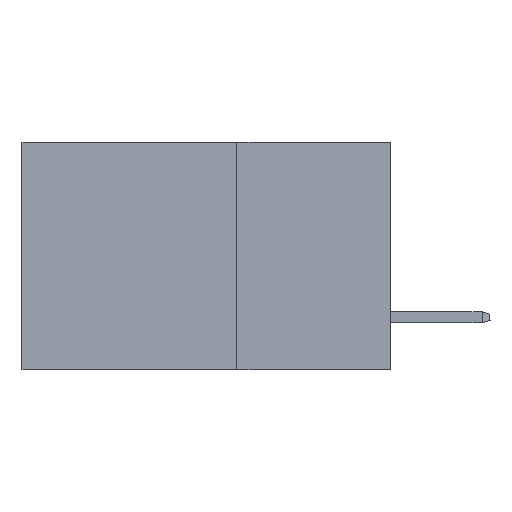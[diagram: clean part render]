
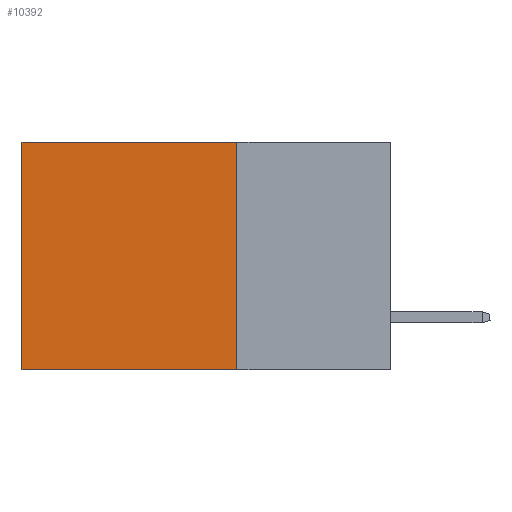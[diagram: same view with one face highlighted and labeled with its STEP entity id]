
A CAD part, left-side view. The second image highlights one B-rep face of the part: STEP entity #10392.
In plain terms, the highlighted planar face has unit normal (-1, 0, 0).
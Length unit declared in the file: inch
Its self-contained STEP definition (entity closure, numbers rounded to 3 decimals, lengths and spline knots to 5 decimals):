
#921 = DIRECTION ( 'NONE',  ( 0., 1., 0. ) ) ;
#1397 = CARTESIAN_POINT ( 'NONE',  ( 0.2875, 0.25, 0. ) ) ;
#1737 = VERTEX_POINT ( 'NONE', #40214 ) ;
#2970 = FACE_OUTER_BOUND ( 'NONE', #36161, .T. ) ;
#3218 = ORIENTED_EDGE ( 'NONE', *, *, #11305, .T. ) ;
#5317 = ORIENTED_EDGE ( 'NONE', *, *, #13658, .F. ) ;
#5333 = PLANE ( 'NONE',  #18214 ) ;
#9111 = VECTOR ( 'NONE', #13002, 39.37008 ) ;
#10392 = ADVANCED_FACE ( 'NONE', ( #2970 ), #5333, .F. ) ;
#10948 = CARTESIAN_POINT ( 'NONE',  ( 0.2875, 0.25, -0.37 ) ) ;
#11305 = EDGE_CURVE ( 'NONE', #42741, #1737, #23768, .T. ) ;
#11705 = CARTESIAN_POINT ( 'NONE',  ( 0.2875, 0.25, 0. ) ) ;
#13002 = DIRECTION ( 'NONE',  ( 0., 0., -1. ) ) ;
#13658 = EDGE_CURVE ( 'NONE', #42741, #17744, #16175, .T. ) ;
#13902 = VECTOR ( 'NONE', #26418, 39.37008 ) ;
#16175 = LINE ( 'NONE', #1397, #43332 ) ;
#17744 = VERTEX_POINT ( 'NONE', #25409 ) ;
#18214 = AXIS2_PLACEMENT_3D ( 'NONE', #11705, #25493, #34989 ) ;
#19635 = LINE ( 'NONE', #10948, #41623 ) ;
#22424 = CARTESIAN_POINT ( 'NONE',  ( 0.2875, 0.6, 0. ) ) ;
#23768 = LINE ( 'NONE', #30101, #13902 ) ;
#23987 = CARTESIAN_POINT ( 'NONE',  ( 0.2875, 0.6, -0.37 ) ) ;
#25061 = CARTESIAN_POINT ( 'NONE',  ( 0.2875, 0.25, 0. ) ) ;
#25409 = CARTESIAN_POINT ( 'NONE',  ( 0.2875, 0.25, -0.37 ) ) ;
#25493 = DIRECTION ( 'NONE',  ( 1., 0., 0. ) ) ;
#26154 = EDGE_CURVE ( 'NONE', #17744, #30456, #19635, .T. ) ;
#26418 = DIRECTION ( 'NONE',  ( 0., 1., 0. ) ) ;
#27875 = LINE ( 'NONE', #22424, #9111 ) ;
#28474 = DIRECTION ( 'NONE',  ( 0., 0., -1. ) ) ;
#30101 = CARTESIAN_POINT ( 'NONE',  ( 0.2875, 0.25, 0. ) ) ;
#30456 = VERTEX_POINT ( 'NONE', #23987 ) ;
#33014 = EDGE_CURVE ( 'NONE', #1737, #30456, #27875, .T. ) ;
#33682 = ORIENTED_EDGE ( 'NONE', *, *, #33014, .T. ) ;
#34989 = DIRECTION ( 'NONE',  ( 0., 0., -1. ) ) ;
#36161 = EDGE_LOOP ( 'NONE', ( #33682, #39701, #5317, #3218 ) ) ;
#39701 = ORIENTED_EDGE ( 'NONE', *, *, #26154, .F. ) ;
#40214 = CARTESIAN_POINT ( 'NONE',  ( 0.2875, 0.6, 0. ) ) ;
#41623 = VECTOR ( 'NONE', #921, 39.37008 ) ;
#42741 = VERTEX_POINT ( 'NONE', #25061 ) ;
#43332 = VECTOR ( 'NONE', #28474, 39.37008 ) ;
